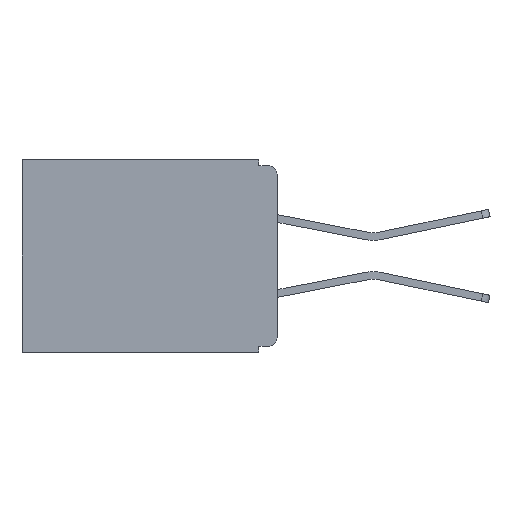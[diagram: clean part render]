
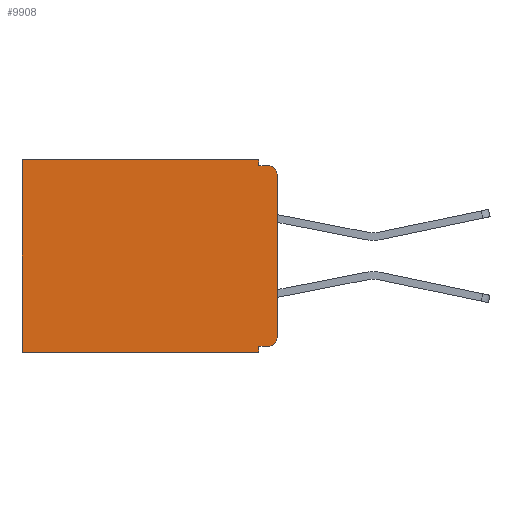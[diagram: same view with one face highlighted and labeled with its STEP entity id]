
A CAD part, left-side view. The second image highlights one B-rep face of the part: STEP entity #9908.
In plain terms, the highlighted planar face has unit normal (-1, 0, 0).
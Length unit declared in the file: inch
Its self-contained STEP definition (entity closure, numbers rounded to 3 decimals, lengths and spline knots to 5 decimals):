
#235 = VERTEX_POINT ( 'NONE', #14706 ) ;
#376 = ORIENTED_EDGE ( 'NONE', *, *, #7720, .F. ) ;
#536 = EDGE_LOOP ( 'NONE', ( #8206, #7818, #376, #20389, #17394, #25511, #3810, #7102, #28060, #5180 ) ) ;
#741 = EDGE_CURVE ( 'NONE', #17141, #11203, #1956, .T. ) ;
#790 = VECTOR ( 'NONE', #16276, 39.37008 ) ;
#797 = CARTESIAN_POINT ( 'NONE',  ( 0.3, 0.031, -0.32 ) ) ;
#1956 = LINE ( 'NONE', #19303, #7194 ) ;
#1984 = DIRECTION ( 'NONE',  ( 0., 0., -1. ) ) ;
#2534 = LINE ( 'NONE', #9439, #21988 ) ;
#2892 = CARTESIAN_POINT ( 'NONE',  ( 0.3, 0.437, 0. ) ) ;
#3034 = CARTESIAN_POINT ( 'NONE',  ( 0.3, 0., -0.33 ) ) ;
#3810 = ORIENTED_EDGE ( 'NONE', *, *, #29744, .F. ) ;
#4086 = DIRECTION ( 'NONE',  ( 1., 0., 0. ) ) ;
#4812 = DIRECTION ( 'NONE',  ( 0., 0., -1. ) ) ;
#5180 = ORIENTED_EDGE ( 'NONE', *, *, #9624, .T. ) ;
#5524 = EDGE_CURVE ( 'NONE', #25874, #9342, #32028, .T. ) ;
#6371 = LINE ( 'NONE', #22522, #25643 ) ;
#6590 = CARTESIAN_POINT ( 'NONE',  ( 0.3, 0., -0.33 ) ) ;
#6604 = CARTESIAN_POINT ( 'NONE',  ( 0.3, 0.031, 0. ) ) ;
#7102 = ORIENTED_EDGE ( 'NONE', *, *, #20550, .F. ) ;
#7194 = VECTOR ( 'NONE', #1984, 39.37008 ) ;
#7674 = CARTESIAN_POINT ( 'NONE',  ( 0.3, 0., -0.305 ) ) ;
#7720 = EDGE_CURVE ( 'NONE', #24746, #9342, #15425, .T. ) ;
#7818 = ORIENTED_EDGE ( 'NONE', *, *, #5524, .T. ) ;
#8193 = CARTESIAN_POINT ( 'NONE',  ( 0.3, 0.015, -0.305 ) ) ;
#8206 = ORIENTED_EDGE ( 'NONE', *, *, #13891, .F. ) ;
#8663 = VECTOR ( 'NONE', #21846, 39.37008 ) ;
#9064 = LINE ( 'NONE', #3034, #14251 ) ;
#9321 = EDGE_CURVE ( 'NONE', #18686, #17141, #2534, .T. ) ;
#9342 = VERTEX_POINT ( 'NONE', #24550 ) ;
#9439 = CARTESIAN_POINT ( 'NONE',  ( 0.3, 0., 0. ) ) ;
#9624 = EDGE_CURVE ( 'NONE', #235, #12026, #25548, .T. ) ;
#9648 = DIRECTION ( 'NONE',  ( 0., 1., 0. ) ) ;
#9908 = ADVANCED_FACE ( 'NONE', ( #17808 ), #16860, .F. ) ;
#10717 = DIRECTION ( 'NONE',  ( 0., 0., -1. ) ) ;
#11203 = VERTEX_POINT ( 'NONE', #19395 ) ;
#11980 = DIRECTION ( 'NONE',  ( 0., 1., 0. ) ) ;
#12026 = VERTEX_POINT ( 'NONE', #7674 ) ;
#12371 = LINE ( 'NONE', #6604, #15166 ) ;
#13704 = CARTESIAN_POINT ( 'NONE',  ( 0.3, 0.031, -0.33 ) ) ;
#13891 = EDGE_CURVE ( 'NONE', #25874, #12026, #6371, .T. ) ;
#13956 = CARTESIAN_POINT ( 'NONE',  ( 0.3, 0.031, 0. ) ) ;
#14251 = VECTOR ( 'NONE', #23285, 39.37008 ) ;
#14253 = DIRECTION ( 'NONE',  ( -1., 0., 0. ) ) ;
#14706 = CARTESIAN_POINT ( 'NONE',  ( 0.3, 0.015, -0.32 ) ) ;
#15045 = VERTEX_POINT ( 'NONE', #17130 ) ;
#15166 = VECTOR ( 'NONE', #26675, 39.37008 ) ;
#15425 = LINE ( 'NONE', #21176, #8663 ) ;
#16219 = DIRECTION ( 'NONE',  ( 0., 0., -1. ) ) ;
#16276 = DIRECTION ( 'NONE',  ( 0., 0., -1. ) ) ;
#16860 = PLANE ( 'NONE',  #25730 ) ;
#17130 = CARTESIAN_POINT ( 'NONE',  ( 0.3, 0.031, -0.33 ) ) ;
#17141 = VERTEX_POINT ( 'NONE', #2892 ) ;
#17394 = ORIENTED_EDGE ( 'NONE', *, *, #9321, .T. ) ;
#17808 = FACE_OUTER_BOUND ( 'NONE', #536, .T. ) ;
#18686 = VERTEX_POINT ( 'NONE', #13956 ) ;
#19303 = CARTESIAN_POINT ( 'NONE',  ( 0.3, 0.437, -0.33 ) ) ;
#19395 = CARTESIAN_POINT ( 'NONE',  ( 0.3, 0.437, -0.33 ) ) ;
#19717 = CARTESIAN_POINT ( 'NONE',  ( 0.3, 0., -0.32 ) ) ;
#20389 = ORIENTED_EDGE ( 'NONE', *, *, #27132, .F. ) ;
#20550 = EDGE_CURVE ( 'NONE', #26331, #15045, #21078, .T. ) ;
#21078 = LINE ( 'NONE', #13704, #790 ) ;
#21176 = CARTESIAN_POINT ( 'NONE',  ( 0.3, 0., -0.01 ) ) ;
#21586 = VECTOR ( 'NONE', #9648, 39.37008 ) ;
#21711 = AXIS2_PLACEMENT_3D ( 'NONE', #26749, #14253, #16219 ) ;
#21826 = DIRECTION ( 'NONE',  ( 0., 0., -1. ) ) ;
#21846 = DIRECTION ( 'NONE',  ( 0., -1., 0. ) ) ;
#21988 = VECTOR ( 'NONE', #11980, 39.37008 ) ;
#22360 = LINE ( 'NONE', #19717, #21586 ) ;
#22522 = CARTESIAN_POINT ( 'NONE',  ( 0.3, 0., -0.33 ) ) ;
#23025 = AXIS2_PLACEMENT_3D ( 'NONE', #8193, #25728, #10717 ) ;
#23285 = DIRECTION ( 'NONE',  ( 0., 1., 0. ) ) ;
#24550 = CARTESIAN_POINT ( 'NONE',  ( 0.3, 0.015, -0.01 ) ) ;
#24746 = VERTEX_POINT ( 'NONE', #26730 ) ;
#25511 = ORIENTED_EDGE ( 'NONE', *, *, #741, .T. ) ;
#25548 = CIRCLE ( 'NONE', #23025, 0.015 ) ;
#25643 = VECTOR ( 'NONE', #4812, 39.37008 ) ;
#25728 = DIRECTION ( 'NONE',  ( -1., 0., 0. ) ) ;
#25730 = AXIS2_PLACEMENT_3D ( 'NONE', #6590, #4086, #21826 ) ;
#25874 = VERTEX_POINT ( 'NONE', #30941 ) ;
#26331 = VERTEX_POINT ( 'NONE', #797 ) ;
#26675 = DIRECTION ( 'NONE',  ( 0., 0., -1. ) ) ;
#26730 = CARTESIAN_POINT ( 'NONE',  ( 0.3, 0.031, -0.01 ) ) ;
#26749 = CARTESIAN_POINT ( 'NONE',  ( 0.3, 0.015, -0.025 ) ) ;
#27132 = EDGE_CURVE ( 'NONE', #18686, #24746, #12371, .T. ) ;
#28060 = ORIENTED_EDGE ( 'NONE', *, *, #30573, .F. ) ;
#29744 = EDGE_CURVE ( 'NONE', #15045, #11203, #9064, .T. ) ;
#30573 = EDGE_CURVE ( 'NONE', #235, #26331, #22360, .T. ) ;
#30941 = CARTESIAN_POINT ( 'NONE',  ( 0.3, 0., -0.025 ) ) ;
#32028 = CIRCLE ( 'NONE', #21711, 0.015 ) ;
